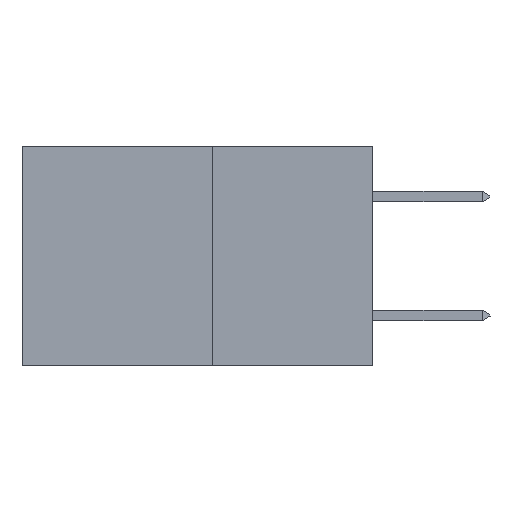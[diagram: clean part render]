
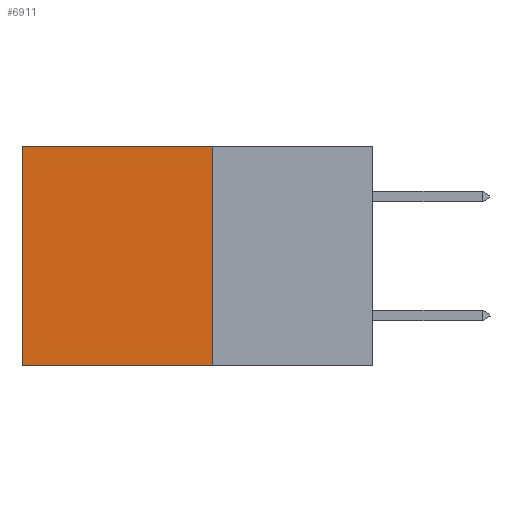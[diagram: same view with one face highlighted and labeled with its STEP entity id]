
A CAD part, left-side view. The second image highlights one B-rep face of the part: STEP entity #6911.
In plain terms, the highlighted planar face has unit normal (-1, 0, 0).
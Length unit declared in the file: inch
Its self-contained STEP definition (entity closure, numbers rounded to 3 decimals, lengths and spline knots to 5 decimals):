
#294 = VECTOR ( 'NONE', #4884, 39.37008 ) ;
#797 = CARTESIAN_POINT ( 'NONE',  ( 0.277, 0.27, 0. ) ) ;
#1289 = EDGE_CURVE ( 'NONE', #4778, #1700, #7183, .T. ) ;
#1700 = VERTEX_POINT ( 'NONE', #7776 ) ;
#1914 = LINE ( 'NONE', #7162, #6211 ) ;
#2029 = DIRECTION ( 'NONE',  ( 0., 0., -1. ) ) ;
#2055 = EDGE_CURVE ( 'NONE', #2822, #1700, #1914, .T. ) ;
#2822 = VERTEX_POINT ( 'NONE', #6918 ) ;
#3335 = ORIENTED_EDGE ( 'NONE', *, *, #7743, .T. ) ;
#3958 = EDGE_CURVE ( 'NONE', #6172, #4778, #8842, .T. ) ;
#4086 = VECTOR ( 'NONE', #9636, 39.37008 ) ;
#4746 = DIRECTION ( 'NONE',  ( 0., 0., -1. ) ) ;
#4778 = VERTEX_POINT ( 'NONE', #6530 ) ;
#4884 = DIRECTION ( 'NONE',  ( 0., 1., 0. ) ) ;
#5708 = ORIENTED_EDGE ( 'NONE', *, *, #1289, .F. ) ;
#6172 = VERTEX_POINT ( 'NONE', #797 ) ;
#6211 = VECTOR ( 'NONE', #7140, 39.37008 ) ;
#6389 = LINE ( 'NONE', #11007, #4086 ) ;
#6470 = AXIS2_PLACEMENT_3D ( 'NONE', #10686, #7778, #2029 ) ;
#6530 = CARTESIAN_POINT ( 'NONE',  ( 0.277, 0.27, -0.37 ) ) ;
#6575 = ORIENTED_EDGE ( 'NONE', *, *, #2055, .T. ) ;
#6911 = ADVANCED_FACE ( 'NONE', ( #10420 ), #8082, .F. ) ;
#6918 = CARTESIAN_POINT ( 'NONE',  ( 0.277, 0.59, 0. ) ) ;
#7021 = ORIENTED_EDGE ( 'NONE', *, *, #3958, .F. ) ;
#7140 = DIRECTION ( 'NONE',  ( 0., 0., -1. ) ) ;
#7162 = CARTESIAN_POINT ( 'NONE',  ( 0.277, 0.59, -0.37 ) ) ;
#7183 = LINE ( 'NONE', #10249, #294 ) ;
#7743 = EDGE_CURVE ( 'NONE', #6172, #2822, #6389, .T. ) ;
#7776 = CARTESIAN_POINT ( 'NONE',  ( 0.277, 0.59, -0.37 ) ) ;
#7778 = DIRECTION ( 'NONE',  ( 1., 0., 0. ) ) ;
#8054 = VECTOR ( 'NONE', #4746, 39.37008 ) ;
#8082 = PLANE ( 'NONE',  #6470 ) ;
#8367 = CARTESIAN_POINT ( 'NONE',  ( 0.277, 0.27, -0.37 ) ) ;
#8842 = LINE ( 'NONE', #8367, #8054 ) ;
#9045 = EDGE_LOOP ( 'NONE', ( #6575, #5708, #7021, #3335 ) ) ;
#9636 = DIRECTION ( 'NONE',  ( 0., 1., 0. ) ) ;
#10249 = CARTESIAN_POINT ( 'NONE',  ( 0.277, 0.27, -0.37 ) ) ;
#10420 = FACE_OUTER_BOUND ( 'NONE', #9045, .T. ) ;
#10686 = CARTESIAN_POINT ( 'NONE',  ( 0.277, 0.27, -0.37 ) ) ;
#11007 = CARTESIAN_POINT ( 'NONE',  ( 0.277, 0.27, 0. ) ) ;
